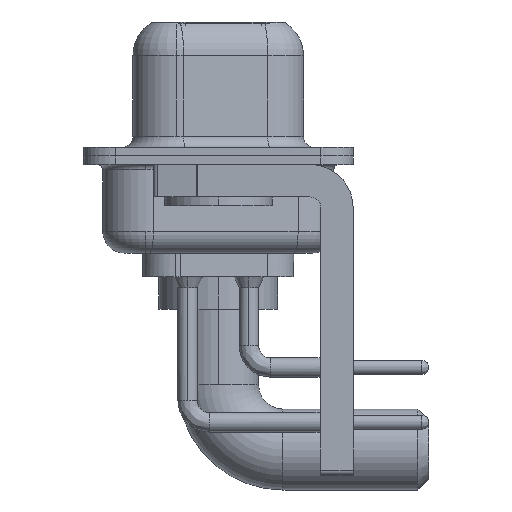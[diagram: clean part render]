
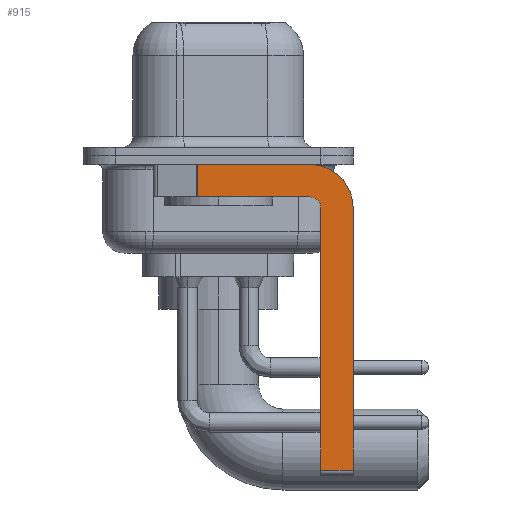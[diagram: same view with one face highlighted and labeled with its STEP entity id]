
A CAD part, left-side view. The second image highlights one B-rep face of the part: STEP entity #915.
In plain terms, the highlighted planar face has unit normal (-1, 0, 0).
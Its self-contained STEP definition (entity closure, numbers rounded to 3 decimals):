
#29 = VERTEX_POINT ( 'NONE', #4088 ) ;
#45 = VERTEX_POINT ( 'NONE', #6771 ) ;
#250 = CARTESIAN_POINT ( 'NONE',  ( -2.9, -6.25, -2.4 ) ) ;
#337 = ORIENTED_EDGE ( 'NONE', *, *, #18460, .T. ) ;
#466 = DIRECTION ( 'NONE',  ( 0., 0., -1. ) ) ;
#471 = EDGE_CURVE ( 'NONE', #18691, #6713, #16053, .T. ) ;
#628 = DIRECTION ( 'NONE',  ( -1., 0., 0. ) ) ;
#915 = ADVANCED_FACE ( 'NONE', ( #5600 ), #2739, .F. ) ;
#1251 = AXIS2_PLACEMENT_3D ( 'NONE', #18956, #11594, #10129 ) ;
#1394 = VECTOR ( 'NONE', #11917, 1000. ) ;
#1854 = EDGE_CURVE ( 'NONE', #7694, #2399, #3443, .T. ) ;
#2112 = ORIENTED_EDGE ( 'NONE', *, *, #5587, .F. ) ;
#2157 = CARTESIAN_POINT ( 'NONE',  ( -2.9, 3., -0.4 ) ) ;
#2210 = EDGE_CURVE ( 'NONE', #17769, #29, #11188, .T. ) ;
#2399 = VERTEX_POINT ( 'NONE', #4004 ) ;
#2719 = ORIENTED_EDGE ( 'NONE', *, *, #5858, .F. ) ;
#2739 = PLANE ( 'NONE',  #1251 ) ;
#3223 = ORIENTED_EDGE ( 'NONE', *, *, #15100, .T. ) ;
#3438 = CARTESIAN_POINT ( 'NONE',  ( -2.9, -4.25, -1.9 ) ) ;
#3443 = LINE ( 'NONE', #2157, #17926 ) ;
#3660 = EDGE_LOOP ( 'NONE', ( #9212, #337, #4433, #9377, #2719, #3223, #6996, #2112 ) ) ;
#3820 = VECTOR ( 'NONE', #466, 1000. ) ;
#4004 = CARTESIAN_POINT ( 'NONE',  ( -2.9, -4.25, -0.4 ) ) ;
#4081 = CARTESIAN_POINT ( 'NONE',  ( -2.9, -4.25, -2.4 ) ) ;
#4088 = CARTESIAN_POINT ( 'NONE',  ( -2.9, -6.25, -14.55 ) ) ;
#4433 = ORIENTED_EDGE ( 'NONE', *, *, #471, .F. ) ;
#4435 = LINE ( 'NONE', #19367, #1394 ) ;
#5317 = DIRECTION ( 'NONE',  ( 0., 0., 1. ) ) ;
#5587 = EDGE_CURVE ( 'NONE', #2399, #17769, #17497, .T. ) ;
#5600 = FACE_OUTER_BOUND ( 'NONE', #3660, .T. ) ;
#5858 = EDGE_CURVE ( 'NONE', #9918, #45, #17419, .T. ) ;
#6713 = VERTEX_POINT ( 'NONE', #15022 ) ;
#6771 = CARTESIAN_POINT ( 'NONE',  ( -2.9, -4.75, -2.4 ) ) ;
#6996 = ORIENTED_EDGE ( 'NONE', *, *, #2210, .F. ) ;
#7304 = CARTESIAN_POINT ( 'NONE',  ( -2.9, -4.25, -14.55 ) ) ;
#7499 = CARTESIAN_POINT ( 'NONE',  ( -2.9, 0.978, -0.4 ) ) ;
#7694 = VERTEX_POINT ( 'NONE', #7499 ) ;
#8622 = EDGE_CURVE ( 'NONE', #45, #18691, #10282, .T. ) ;
#9031 = AXIS2_PLACEMENT_3D ( 'NONE', #4081, #14419, #14809 ) ;
#9212 = ORIENTED_EDGE ( 'NONE', *, *, #1854, .F. ) ;
#9377 = ORIENTED_EDGE ( 'NONE', *, *, #8622, .F. ) ;
#9918 = VERTEX_POINT ( 'NONE', #15429 ) ;
#10129 = DIRECTION ( 'NONE',  ( 0., 0., -1. ) ) ;
#10253 = LINE ( 'NONE', #7304, #17981 ) ;
#10282 = CIRCLE ( 'NONE', #15929, 0.5 ) ;
#11124 = DIRECTION ( 'NONE',  ( 0., -1., 0. ) ) ;
#11188 = LINE ( 'NONE', #13759, #3820 ) ;
#11594 = DIRECTION ( 'NONE',  ( 1., 0., 0. ) ) ;
#11917 = DIRECTION ( 'NONE',  ( 0., 0., -1. ) ) ;
#13193 = DIRECTION ( 'NONE',  ( 0., -1., 0. ) ) ;
#13759 = CARTESIAN_POINT ( 'NONE',  ( -2.9, -6.25, -2.4 ) ) ;
#14026 = CARTESIAN_POINT ( 'NONE',  ( -2.9, -4.25, -2.4 ) ) ;
#14419 = DIRECTION ( 'NONE',  ( 1., 0., 0. ) ) ;
#14581 = CARTESIAN_POINT ( 'NONE',  ( -2.9, -4.25, -1.9 ) ) ;
#14809 = DIRECTION ( 'NONE',  ( 0., 0., -1. ) ) ;
#15022 = CARTESIAN_POINT ( 'NONE',  ( -2.9, 0.978, -1.9 ) ) ;
#15100 = EDGE_CURVE ( 'NONE', #9918, #29, #10253, .T. ) ;
#15429 = CARTESIAN_POINT ( 'NONE',  ( -2.9, -4.75, -14.55 ) ) ;
#15929 = AXIS2_PLACEMENT_3D ( 'NONE', #14026, #628, #17452 ) ;
#15959 = VECTOR ( 'NONE', #17428, 1000. ) ;
#16053 = LINE ( 'NONE', #14581, #15959 ) ;
#16548 = VECTOR ( 'NONE', #5317, 1000. ) ;
#17419 = LINE ( 'NONE', #19069, #16548 ) ;
#17428 = DIRECTION ( 'NONE',  ( 0., 1., 0. ) ) ;
#17452 = DIRECTION ( 'NONE',  ( 0., 0., 1. ) ) ;
#17497 = CIRCLE ( 'NONE', #9031, 2. ) ;
#17769 = VERTEX_POINT ( 'NONE', #250 ) ;
#17926 = VECTOR ( 'NONE', #11124, 1000. ) ;
#17981 = VECTOR ( 'NONE', #13193, 1000. ) ;
#18460 = EDGE_CURVE ( 'NONE', #7694, #6713, #4435, .T. ) ;
#18691 = VERTEX_POINT ( 'NONE', #3438 ) ;
#18956 = CARTESIAN_POINT ( 'NONE',  ( -2.9, -4.25, -2.4 ) ) ;
#19069 = CARTESIAN_POINT ( 'NONE',  ( -2.9, -4.75, -14.8 ) ) ;
#19367 = CARTESIAN_POINT ( 'NONE',  ( -2.9, 0.978, -1.9 ) ) ;
